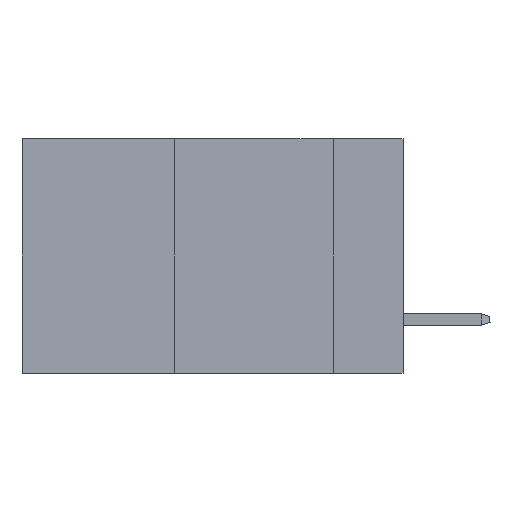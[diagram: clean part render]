
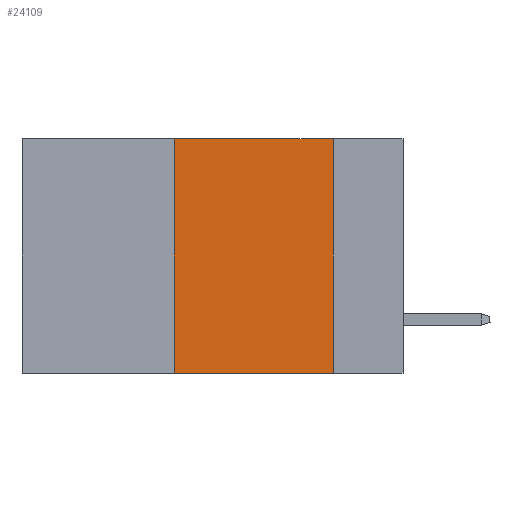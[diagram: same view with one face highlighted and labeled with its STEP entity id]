
A CAD part, left-side view. The second image highlights one B-rep face of the part: STEP entity #24109.
In plain terms, the highlighted planar face has unit normal (-1, 0, 0).
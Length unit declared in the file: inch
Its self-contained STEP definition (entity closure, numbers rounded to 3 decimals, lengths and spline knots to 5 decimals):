
#168 = DIRECTION ( 'NONE',  ( 1., 0., 0. ) ) ;
#239 = EDGE_LOOP ( 'NONE', ( #6738, #10128, #875, #8207 ) ) ;
#875 = ORIENTED_EDGE ( 'NONE', *, *, #7194, .F. ) ;
#1323 = VERTEX_POINT ( 'NONE', #7957 ) ;
#1950 = CARTESIAN_POINT ( 'NONE',  ( 0., 0.11, 0. ) ) ;
#2531 = LINE ( 'NONE', #11238, #10347 ) ;
#4708 = CARTESIAN_POINT ( 'NONE',  ( 0., 0.6, 0. ) ) ;
#4948 = CARTESIAN_POINT ( 'NONE',  ( 0., 0.36, 0. ) ) ;
#6176 = CARTESIAN_POINT ( 'NONE',  ( 0., 0.6, 0. ) ) ;
#6738 = ORIENTED_EDGE ( 'NONE', *, *, #17894, .F. ) ;
#7170 = CARTESIAN_POINT ( 'NONE',  ( 0., 0.11, -0.37 ) ) ;
#7194 = EDGE_CURVE ( 'NONE', #1323, #16953, #15732, .T. ) ;
#7957 = CARTESIAN_POINT ( 'NONE',  ( 0., 0.36, -0.37 ) ) ;
#8207 = ORIENTED_EDGE ( 'NONE', *, *, #13038, .T. ) ;
#8960 = PLANE ( 'NONE',  #22077 ) ;
#9097 = DIRECTION ( 'NONE',  ( 0., -1., 0. ) ) ;
#10128 = ORIENTED_EDGE ( 'NONE', *, *, #14273, .F. ) ;
#10347 = VECTOR ( 'NONE', #9097, 39.37008 ) ;
#10612 = DIRECTION ( 'NONE',  ( 0., 0., -1. ) ) ;
#11238 = CARTESIAN_POINT ( 'NONE',  ( 0., 0.6, -0.37 ) ) ;
#13038 = EDGE_CURVE ( 'NONE', #1323, #22043, #2531, .T. ) ;
#13356 = DIRECTION ( 'NONE',  ( 0., 0., -1. ) ) ;
#14200 = VECTOR ( 'NONE', #22546, 39.37008 ) ;
#14273 = EDGE_CURVE ( 'NONE', #16953, #17870, #16942, .T. ) ;
#15732 = LINE ( 'NONE', #4948, #14200 ) ;
#16942 = LINE ( 'NONE', #6176, #22740 ) ;
#16953 = VERTEX_POINT ( 'NONE', #19825 ) ;
#17870 = VERTEX_POINT ( 'NONE', #23416 ) ;
#17894 = EDGE_CURVE ( 'NONE', #17870, #22043, #21529, .T. ) ;
#18057 = VECTOR ( 'NONE', #10612, 39.37008 ) ;
#19825 = CARTESIAN_POINT ( 'NONE',  ( 0., 0.36, 0. ) ) ;
#21529 = LINE ( 'NONE', #1950, #18057 ) ;
#22043 = VERTEX_POINT ( 'NONE', #7170 ) ;
#22077 = AXIS2_PLACEMENT_3D ( 'NONE', #4708, #168, #13356 ) ;
#22181 = FACE_OUTER_BOUND ( 'NONE', #239, .T. ) ;
#22546 = DIRECTION ( 'NONE',  ( 0., 0., 1. ) ) ;
#22740 = VECTOR ( 'NONE', #27673, 39.37008 ) ;
#23416 = CARTESIAN_POINT ( 'NONE',  ( 0., 0.11, 0. ) ) ;
#24109 = ADVANCED_FACE ( 'NONE', ( #22181 ), #8960, .F. ) ;
#27673 = DIRECTION ( 'NONE',  ( 0., -1., 0. ) ) ;
